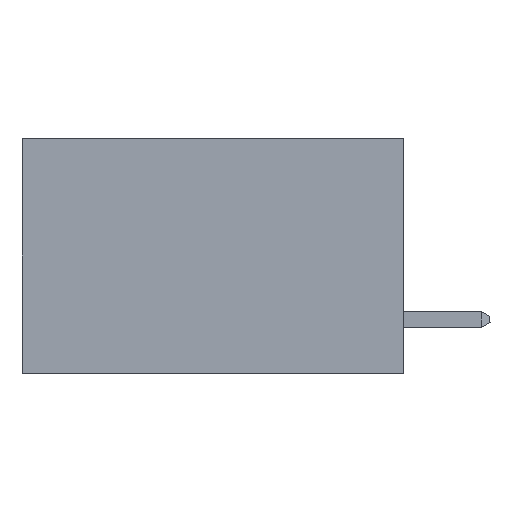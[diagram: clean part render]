
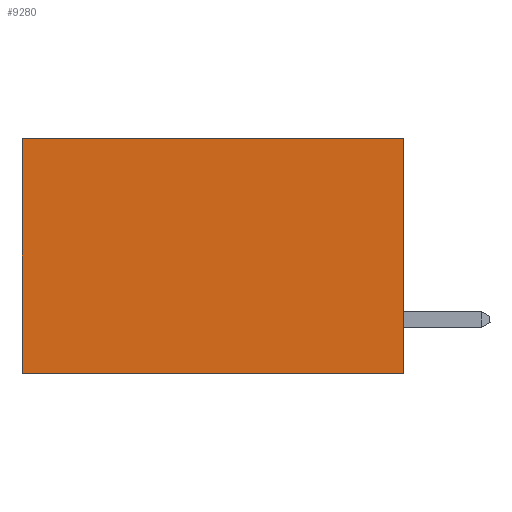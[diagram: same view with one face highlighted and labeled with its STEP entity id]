
A CAD part, left-side view. The second image highlights one B-rep face of the part: STEP entity #9280.
In plain terms, the highlighted planar face has unit normal (-1, 0, 0).
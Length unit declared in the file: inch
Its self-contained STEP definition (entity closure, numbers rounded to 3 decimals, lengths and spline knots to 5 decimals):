
#288 = VECTOR ( 'NONE', #6131, 39.37008 ) ;
#372 = VERTEX_POINT ( 'NONE', #6786 ) ;
#691 = VERTEX_POINT ( 'NONE', #821 ) ;
#821 = CARTESIAN_POINT ( 'NONE',  ( 0.2875, 0.6, -0.37 ) ) ;
#897 = LINE ( 'NONE', #1554, #288 ) ;
#907 = EDGE_LOOP ( 'NONE', ( #7739, #2911, #7029, #2739 ) ) ;
#1047 = CARTESIAN_POINT ( 'NONE',  ( 0.2875, 0., -0.37 ) ) ;
#1097 = DIRECTION ( 'NONE',  ( 1., 0., 0. ) ) ;
#1554 = CARTESIAN_POINT ( 'NONE',  ( 0.2875, 0., 0. ) ) ;
#1769 = EDGE_CURVE ( 'NONE', #4174, #7586, #897, .T. ) ;
#1844 = DIRECTION ( 'NONE',  ( 0., 0., -1. ) ) ;
#2467 = LINE ( 'NONE', #8084, #4474 ) ;
#2486 = PLANE ( 'NONE',  #5237 ) ;
#2520 = CARTESIAN_POINT ( 'NONE',  ( 0.2875, 0., 0. ) ) ;
#2739 = ORIENTED_EDGE ( 'NONE', *, *, #5466, .T. ) ;
#2911 = ORIENTED_EDGE ( 'NONE', *, *, #6680, .F. ) ;
#3170 = DIRECTION ( 'NONE',  ( 0., 1., 0. ) ) ;
#3248 = LINE ( 'NONE', #1047, #4656 ) ;
#4174 = VERTEX_POINT ( 'NONE', #4789 ) ;
#4474 = VECTOR ( 'NONE', #6587, 39.37008 ) ;
#4656 = VECTOR ( 'NONE', #3170, 39.37008 ) ;
#4789 = CARTESIAN_POINT ( 'NONE',  ( 0.2875, 0., 0. ) ) ;
#5237 = AXIS2_PLACEMENT_3D ( 'NONE', #2520, #1097, #1844 ) ;
#5466 = EDGE_CURVE ( 'NONE', #4174, #372, #6596, .T. ) ;
#5495 = CARTESIAN_POINT ( 'NONE',  ( 0.2875, 0., 0. ) ) ;
#6131 = DIRECTION ( 'NONE',  ( 0., 0., -1. ) ) ;
#6301 = EDGE_CURVE ( 'NONE', #372, #691, #2467, .T. ) ;
#6326 = DIRECTION ( 'NONE',  ( 0., 1., 0. ) ) ;
#6352 = FACE_OUTER_BOUND ( 'NONE', #907, .T. ) ;
#6587 = DIRECTION ( 'NONE',  ( 0., 0., -1. ) ) ;
#6596 = LINE ( 'NONE', #5495, #7884 ) ;
#6680 = EDGE_CURVE ( 'NONE', #7586, #691, #3248, .T. ) ;
#6786 = CARTESIAN_POINT ( 'NONE',  ( 0.2875, 0.6, 0. ) ) ;
#7029 = ORIENTED_EDGE ( 'NONE', *, *, #1769, .F. ) ;
#7586 = VERTEX_POINT ( 'NONE', #7965 ) ;
#7739 = ORIENTED_EDGE ( 'NONE', *, *, #6301, .T. ) ;
#7884 = VECTOR ( 'NONE', #6326, 39.37008 ) ;
#7965 = CARTESIAN_POINT ( 'NONE',  ( 0.2875, 0., -0.37 ) ) ;
#8084 = CARTESIAN_POINT ( 'NONE',  ( 0.2875, 0.6, 0. ) ) ;
#9280 = ADVANCED_FACE ( 'NONE', ( #6352 ), #2486, .F. ) ;
